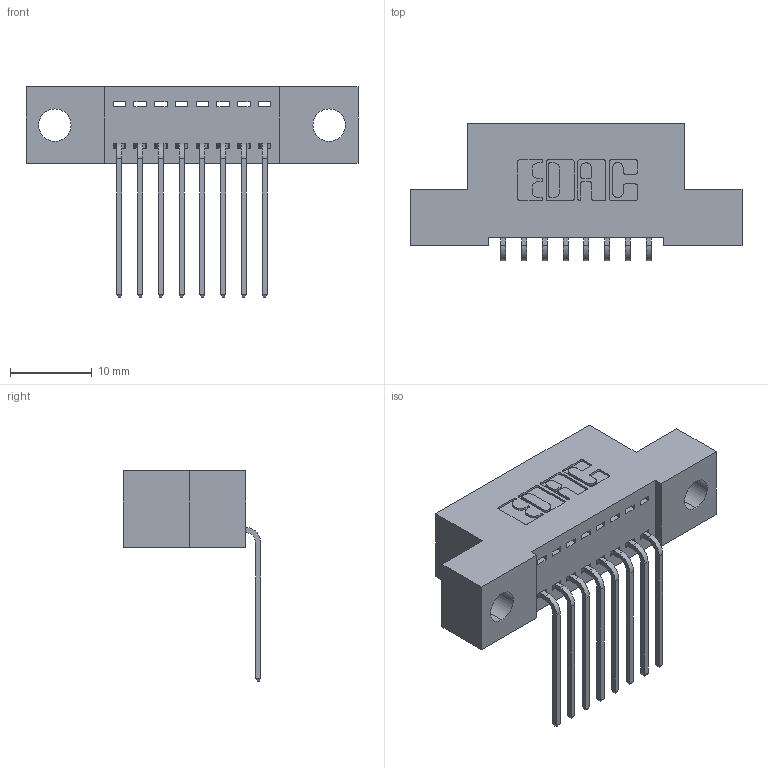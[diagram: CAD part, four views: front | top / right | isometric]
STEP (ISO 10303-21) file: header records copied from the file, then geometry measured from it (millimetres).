
FILE_DESCRIPTION (( 'STEP AP203' ), '1' );
FILE_NAME ('392-008-559-104.STEP', '2019-10-05T00:03:55', ( '' ), ( '' ), 'SwSTEP 2.0', 'SolidWorks 2016', '' );
FILE_SCHEMA (( 'CONFIG_CONTROL_DESIGN' ));
Length unit declared in the file: inch
Products named in the file (3): 392-008-559-104; 342 Part_.156 TH; 345-292-001_558 559 Tail - 1
Assembly tree (9 placements, depth 2):
  392-008-559-104
    342 Part_.156 TH
    345-292-001_558 559 Tail - 1  x8
Bounding box: 40.64 x 16.83 x 25.78 mm (x, y, z)
Volume: 3377.7 mm3; surface area: 4295.3 mm2
Topology: 9 solids, 9 shells, 590 faces, 1755 edges, 1158 vertices
Faces by surface type: plane 418, cylinder 172
Entity records: 9243 total; most frequent: CARTESIAN_POINT 1606, ORIENTED_EDGE 1550, DIRECTION 1423, EDGE_CURVE 775, VECTOR 647, LINE 647, VERTEX_POINT 514, AXIS2_PLACEMENT_3D 388
